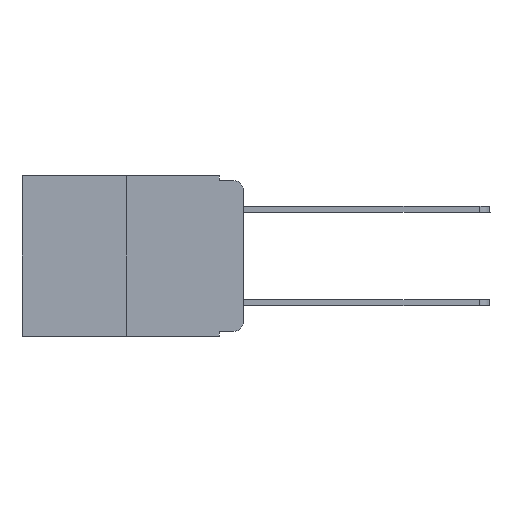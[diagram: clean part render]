
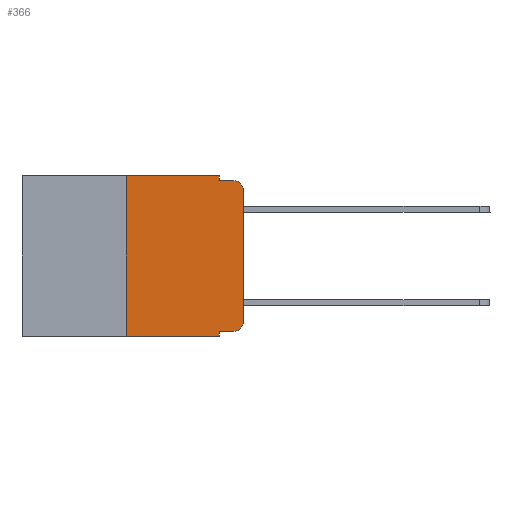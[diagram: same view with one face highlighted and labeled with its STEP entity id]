
A CAD part, left-side view. The second image highlights one B-rep face of the part: STEP entity #366.
In plain terms, the highlighted planar face has unit normal (-1, 0, 0).
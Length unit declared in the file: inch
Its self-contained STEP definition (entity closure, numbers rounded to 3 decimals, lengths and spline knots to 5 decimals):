
#88 = ORIENTED_EDGE ( 'NONE', *, *, #16195, .F. ) ;
#230 = EDGE_CURVE ( 'NONE', #15173, #5304, #14999, .T. ) ;
#366 = ADVANCED_FACE ( 'NONE', ( #16035 ), #20167, .F. ) ;
#371 = DIRECTION ( 'NONE',  ( 0., -1., 0. ) ) ;
#386 = LINE ( 'NONE', #18302, #923 ) ;
#923 = VECTOR ( 'NONE', #16745, 39.37008 ) ;
#1153 = LINE ( 'NONE', #16530, #15263 ) ;
#1428 = ORIENTED_EDGE ( 'NONE', *, *, #7905, .T. ) ;
#1748 = AXIS2_PLACEMENT_3D ( 'NONE', #3940, #2177, #15640 ) ;
#1925 = EDGE_LOOP ( 'NONE', ( #9488, #16568, #14613, #88, #19071, #12887, #5284, #9342, #1428, #12033 ) ) ;
#2055 = DIRECTION ( 'NONE',  ( 0., -1., 0. ) ) ;
#2177 = DIRECTION ( 'NONE',  ( -1., 0., 0. ) ) ;
#2715 = VERTEX_POINT ( 'NONE', #8363 ) ;
#2744 = VECTOR ( 'NONE', #2055, 39.37008 ) ;
#2810 = AXIS2_PLACEMENT_3D ( 'NONE', #9383, #11041, #19293 ) ;
#3440 = DIRECTION ( 'NONE',  ( 1., 0., 0. ) ) ;
#3531 = LINE ( 'NONE', #12246, #2744 ) ;
#3913 = CARTESIAN_POINT ( 'NONE',  ( 0., 0.051, 0. ) ) ;
#3940 = CARTESIAN_POINT ( 'NONE',  ( 0., 0.02, -0.03 ) ) ;
#4150 = EDGE_CURVE ( 'NONE', #12323, #15179, #9220, .T. ) ;
#4294 = CARTESIAN_POINT ( 'NONE',  ( 0., 0., -0.03 ) ) ;
#4403 = VERTEX_POINT ( 'NONE', #9259 ) ;
#4637 = VERTEX_POINT ( 'NONE', #4294 ) ;
#4671 = AXIS2_PLACEMENT_3D ( 'NONE', #13545, #3440, #10049 ) ;
#5284 = ORIENTED_EDGE ( 'NONE', *, *, #6523, .T. ) ;
#5304 = VERTEX_POINT ( 'NONE', #6337 ) ;
#5885 = CARTESIAN_POINT ( 'NONE',  ( 0., 0.02, -0.333 ) ) ;
#6337 = CARTESIAN_POINT ( 'NONE',  ( 0., 0., -0.313 ) ) ;
#6523 = EDGE_CURVE ( 'NONE', #12323, #16462, #11481, .T. ) ;
#6647 = EDGE_CURVE ( 'NONE', #2715, #16929, #10934, .T. ) ;
#7595 = EDGE_CURVE ( 'NONE', #15179, #11569, #386, .T. ) ;
#7905 = EDGE_CURVE ( 'NONE', #4403, #15173, #3531, .T. ) ;
#8363 = CARTESIAN_POINT ( 'NONE',  ( 0., 0.051, -0.01 ) ) ;
#8868 = EDGE_CURVE ( 'NONE', #4403, #16462, #14452, .T. ) ;
#9220 = LINE ( 'NONE', #18094, #17003 ) ;
#9259 = CARTESIAN_POINT ( 'NONE',  ( 0., 0.051, -0.333 ) ) ;
#9342 = ORIENTED_EDGE ( 'NONE', *, *, #8868, .F. ) ;
#9383 = CARTESIAN_POINT ( 'NONE',  ( 0., 0.02, -0.313 ) ) ;
#9488 = ORIENTED_EDGE ( 'NONE', *, *, #10675, .T. ) ;
#9668 = CIRCLE ( 'NONE', #1748, 0.02 ) ;
#9913 = DIRECTION ( 'NONE',  ( 0., 0., 1. ) ) ;
#10049 = DIRECTION ( 'NONE',  ( 0., 0., -1. ) ) ;
#10675 = EDGE_CURVE ( 'NONE', #5304, #4637, #1153, .T. ) ;
#10934 = LINE ( 'NONE', #16960, #17168 ) ;
#11041 = DIRECTION ( 'NONE',  ( -1., 0., 0. ) ) ;
#11481 = LINE ( 'NONE', #17810, #17477 ) ;
#11569 = VERTEX_POINT ( 'NONE', #20679 ) ;
#12033 = ORIENTED_EDGE ( 'NONE', *, *, #230, .T. ) ;
#12246 = CARTESIAN_POINT ( 'NONE',  ( 0., 0.051, -0.333 ) ) ;
#12323 = VERTEX_POINT ( 'NONE', #18115 ) ;
#12419 = DIRECTION ( 'NONE',  ( 0., 0., -1. ) ) ;
#12887 = ORIENTED_EDGE ( 'NONE', *, *, #4150, .F. ) ;
#13071 = CARTESIAN_POINT ( 'NONE',  ( 0., 0.051, -0.343 ) ) ;
#13243 = LINE ( 'NONE', #3913, #15040 ) ;
#13273 = DIRECTION ( 'NONE',  ( 0., -1., 0. ) ) ;
#13545 = CARTESIAN_POINT ( 'NONE',  ( 0., 0.473, 0. ) ) ;
#14189 = VECTOR ( 'NONE', #16201, 39.37008 ) ;
#14341 = CARTESIAN_POINT ( 'NONE',  ( 0., 0.25, 0. ) ) ;
#14452 = LINE ( 'NONE', #19565, #14189 ) ;
#14605 = EDGE_CURVE ( 'NONE', #4637, #16929, #9668, .T. ) ;
#14613 = ORIENTED_EDGE ( 'NONE', *, *, #6647, .F. ) ;
#14999 = CIRCLE ( 'NONE', #2810, 0.02 ) ;
#15040 = VECTOR ( 'NONE', #12419, 39.37008 ) ;
#15173 = VERTEX_POINT ( 'NONE', #5885 ) ;
#15179 = VERTEX_POINT ( 'NONE', #14341 ) ;
#15263 = VECTOR ( 'NONE', #9913, 39.37008 ) ;
#15640 = DIRECTION ( 'NONE',  ( 0., 0., -1. ) ) ;
#16035 = FACE_OUTER_BOUND ( 'NONE', #1925, .T. ) ;
#16195 = EDGE_CURVE ( 'NONE', #11569, #2715, #13243, .T. ) ;
#16201 = DIRECTION ( 'NONE',  ( 0., 0., -1. ) ) ;
#16462 = VERTEX_POINT ( 'NONE', #13071 ) ;
#16530 = CARTESIAN_POINT ( 'NONE',  ( 0., 0., 0. ) ) ;
#16568 = ORIENTED_EDGE ( 'NONE', *, *, #14605, .T. ) ;
#16745 = DIRECTION ( 'NONE',  ( 0., -1., 0. ) ) ;
#16929 = VERTEX_POINT ( 'NONE', #20745 ) ;
#16960 = CARTESIAN_POINT ( 'NONE',  ( 0., 0.051, -0.01 ) ) ;
#17003 = VECTOR ( 'NONE', #19760, 39.37008 ) ;
#17168 = VECTOR ( 'NONE', #371, 39.37008 ) ;
#17477 = VECTOR ( 'NONE', #13273, 39.37008 ) ;
#17810 = CARTESIAN_POINT ( 'NONE',  ( 0., 0.473, -0.343 ) ) ;
#18094 = CARTESIAN_POINT ( 'NONE',  ( 0., 0.25, 0. ) ) ;
#18115 = CARTESIAN_POINT ( 'NONE',  ( 0., 0.25, -0.343 ) ) ;
#18302 = CARTESIAN_POINT ( 'NONE',  ( 0., 0.473, 0. ) ) ;
#19071 = ORIENTED_EDGE ( 'NONE', *, *, #7595, .F. ) ;
#19293 = DIRECTION ( 'NONE',  ( 0., 0., -1. ) ) ;
#19565 = CARTESIAN_POINT ( 'NONE',  ( 0., 0.051, 0. ) ) ;
#19760 = DIRECTION ( 'NONE',  ( 0., 0., 1. ) ) ;
#20167 = PLANE ( 'NONE',  #4671 ) ;
#20679 = CARTESIAN_POINT ( 'NONE',  ( 0., 0.051, 0. ) ) ;
#20745 = CARTESIAN_POINT ( 'NONE',  ( 0., 0.02, -0.01 ) ) ;
